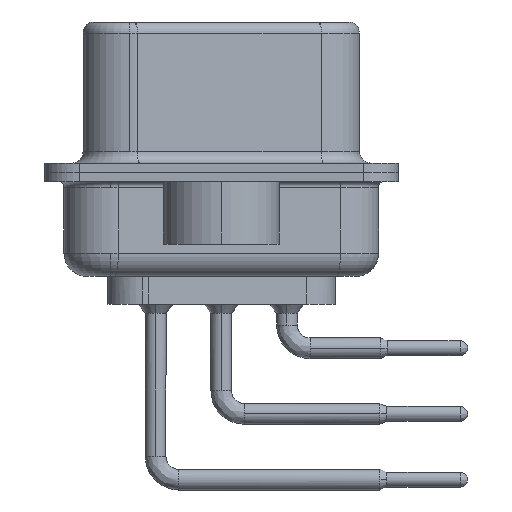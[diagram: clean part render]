
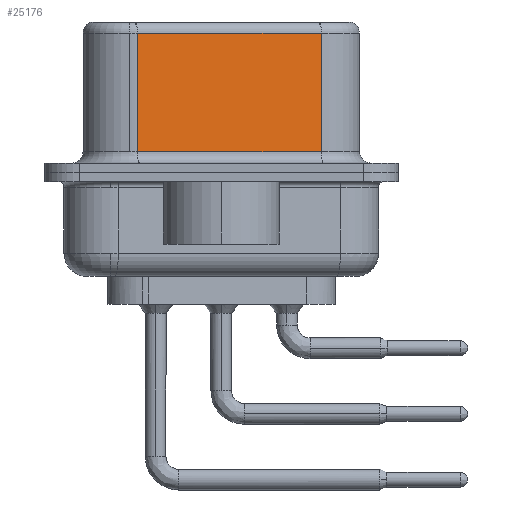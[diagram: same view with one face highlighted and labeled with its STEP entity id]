
A CAD part, left-side view. The second image highlights one B-rep face of the part: STEP entity #25176.
In plain terms, the highlighted planar face has unit normal (-0.985, -0.174, 0).
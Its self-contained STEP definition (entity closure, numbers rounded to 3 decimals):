
#165 = FACE_OUTER_BOUND ( 'NONE', #30792, .T. ) ;
#514 = ORIENTED_EDGE ( 'NONE', *, *, #31418, .F. ) ;
#1107 = DIRECTION ( 'NONE',  ( 0.985, 0.174, 0. ) ) ;
#2486 = DIRECTION ( 'NONE',  ( 0.174, -0.985, 0. ) ) ;
#4632 = VERTEX_POINT ( 'NONE', #8743 ) ;
#5113 = DIRECTION ( 'NONE',  ( 0., 0., -1. ) ) ;
#6438 = VECTOR ( 'NONE', #2486, 1000. ) ;
#6719 = VECTOR ( 'NONE', #5113, 1000. ) ;
#6747 = CARTESIAN_POINT ( 'NONE',  ( 5.132, -4.322, 6.52 ) ) ;
#7227 = LINE ( 'NONE', #36273, #36823 ) ;
#8743 = CARTESIAN_POINT ( 'NONE',  ( 3.73, 3.628, 0.9 ) ) ;
#9187 = EDGE_CURVE ( 'NONE', #17926, #33236, #23743, .T. ) ;
#13583 = LINE ( 'NONE', #25190, #6719 ) ;
#14473 = CARTESIAN_POINT ( 'NONE',  ( 5.132, -4.322, 6.02 ) ) ;
#17139 = EDGE_CURVE ( 'NONE', #4632, #35224, #21753, .T. ) ;
#17926 = VERTEX_POINT ( 'NONE', #14473 ) ;
#20418 = ORIENTED_EDGE ( 'NONE', *, *, #28225, .T. ) ;
#21226 = DIRECTION ( 'NONE',  ( -0.174, 0.985, 0. ) ) ;
#21753 = LINE ( 'NONE', #36819, #6438 ) ;
#21988 = CARTESIAN_POINT ( 'NONE',  ( 3.73, 3.628, 6.02 ) ) ;
#22863 = VECTOR ( 'NONE', #34160, 1000. ) ;
#23743 = LINE ( 'NONE', #28332, #22863 ) ;
#24186 = ORIENTED_EDGE ( 'NONE', *, *, #9187, .T. ) ;
#24924 = DIRECTION ( 'NONE',  ( 0., 0., -1. ) ) ;
#25176 = ADVANCED_FACE ( 'NONE', ( #165 ), #35452, .F. ) ;
#25190 = CARTESIAN_POINT ( 'NONE',  ( 3.73, 3.628, 6.52 ) ) ;
#28017 = ORIENTED_EDGE ( 'NONE', *, *, #17139, .T. ) ;
#28225 = EDGE_CURVE ( 'NONE', #33236, #4632, #13583, .T. ) ;
#28332 = CARTESIAN_POINT ( 'NONE',  ( 5.132, -4.322, 6.02 ) ) ;
#29363 = CARTESIAN_POINT ( 'NONE',  ( 5.132, -4.322, 0.9 ) ) ;
#30792 = EDGE_LOOP ( 'NONE', ( #514, #24186, #20418, #28017 ) ) ;
#31418 = EDGE_CURVE ( 'NONE', #17926, #35224, #7227, .T. ) ;
#31721 = AXIS2_PLACEMENT_3D ( 'NONE', #6747, #1107, #21226 ) ;
#33236 = VERTEX_POINT ( 'NONE', #21988 ) ;
#34160 = DIRECTION ( 'NONE',  ( -0.174, 0.985, 0. ) ) ;
#35224 = VERTEX_POINT ( 'NONE', #29363 ) ;
#35452 = PLANE ( 'NONE',  #31721 ) ;
#36273 = CARTESIAN_POINT ( 'NONE',  ( 5.132, -4.322, 6.52 ) ) ;
#36819 = CARTESIAN_POINT ( 'NONE',  ( 5.132, -4.322, 0.9 ) ) ;
#36823 = VECTOR ( 'NONE', #24924, 1000. ) ;
